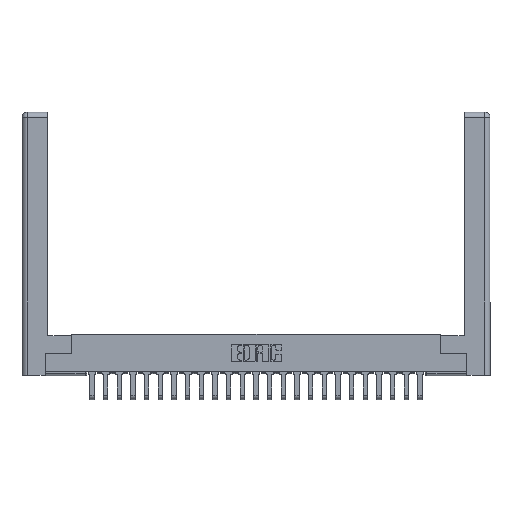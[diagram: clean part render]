
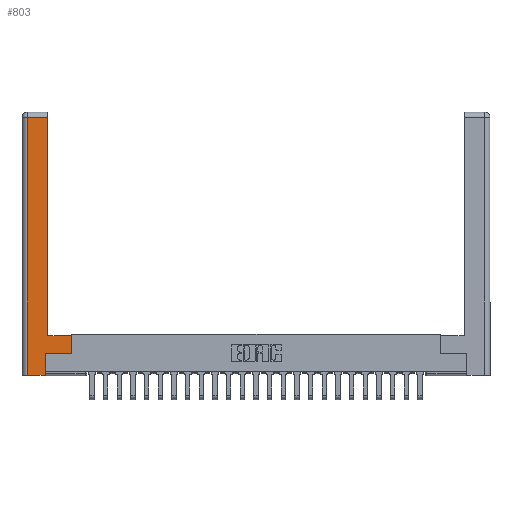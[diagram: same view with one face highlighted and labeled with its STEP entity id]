
A CAD part, top view. The second image highlights one B-rep face of the part: STEP entity #803.
In plain terms, the highlighted planar face has unit normal (0, 0, 1).
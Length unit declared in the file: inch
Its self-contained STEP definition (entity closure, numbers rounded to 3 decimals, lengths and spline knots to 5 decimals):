
#139 = LINE ( 'NONE', #9183, #15880 ) ;
#279 = DIRECTION ( 'NONE',  ( 1., 0., 0. ) ) ;
#803 = ADVANCED_FACE ( 'NONE', ( #17523 ), #23746, .F. ) ;
#818 = CARTESIAN_POINT ( 'NONE',  ( 0.295, 0.45, 0. ) ) ;
#1578 = EDGE_CURVE ( 'NONE', #24801, #14544, #23377, .T. ) ;
#2688 = CARTESIAN_POINT ( 'NONE',  ( 0.565, 0.245, 0. ) ) ;
#2807 = ORIENTED_EDGE ( 'NONE', *, *, #1578, .T. ) ;
#3940 = CARTESIAN_POINT ( 'NONE',  ( 0.0615, 2.94, 0. ) ) ;
#4100 = ORIENTED_EDGE ( 'NONE', *, *, #19604, .T. ) ;
#4155 = CARTESIAN_POINT ( 'NONE',  ( 0.295, 2.94, 0. ) ) ;
#4792 = VERTEX_POINT ( 'NONE', #4155 ) ;
#4798 = VECTOR ( 'NONE', #12545, 39.37008 ) ;
#4860 = DIRECTION ( 'NONE',  ( 0., -1., 0. ) ) ;
#5000 = EDGE_CURVE ( 'NONE', #12074, #17344, #24607, .T. ) ;
#5079 = VECTOR ( 'NONE', #25172, 39.37008 ) ;
#6153 = DIRECTION ( 'NONE',  ( -1., 0., 0. ) ) ;
#6248 = EDGE_CURVE ( 'NONE', #17344, #8954, #139, .T. ) ;
#6306 = ORIENTED_EDGE ( 'NONE', *, *, #8694, .T. ) ;
#6755 = VERTEX_POINT ( 'NONE', #818 ) ;
#7796 = LINE ( 'NONE', #11985, #20072 ) ;
#8694 = EDGE_CURVE ( 'NONE', #4792, #12074, #10130, .T. ) ;
#8954 = VERTEX_POINT ( 'NONE', #11681 ) ;
#8993 = EDGE_LOOP ( 'NONE', ( #12069, #6306, #12452, #15096, #4100, #24421, #2807, #22896 ) ) ;
#9183 = CARTESIAN_POINT ( 'NONE',  ( 0.265, 0., 0. ) ) ;
#10130 = LINE ( 'NONE', #3940, #23446 ) ;
#10365 = EDGE_CURVE ( 'NONE', #14544, #6755, #12393, .T. ) ;
#10383 = CARTESIAN_POINT ( 'NONE',  ( 0.295, 0.45, 0. ) ) ;
#11309 = CARTESIAN_POINT ( 'NONE',  ( 0.565, 0.45, 0. ) ) ;
#11681 = CARTESIAN_POINT ( 'NONE',  ( 0.265, 0., 0. ) ) ;
#11730 = DIRECTION ( 'NONE',  ( 0., 1., 0. ) ) ;
#11985 = CARTESIAN_POINT ( 'NONE',  ( 0.565, 0.245, 0. ) ) ;
#12069 = ORIENTED_EDGE ( 'NONE', *, *, #17331, .T. ) ;
#12074 = VERTEX_POINT ( 'NONE', #13469 ) ;
#12393 = LINE ( 'NONE', #10383, #4798 ) ;
#12452 = ORIENTED_EDGE ( 'NONE', *, *, #5000, .T. ) ;
#12545 = DIRECTION ( 'NONE',  ( -1., 0., 0. ) ) ;
#13469 = CARTESIAN_POINT ( 'NONE',  ( 0.0615, 2.94, 0. ) ) ;
#13739 = LINE ( 'NONE', #18353, #25295 ) ;
#13994 = EDGE_CURVE ( 'NONE', #18421, #24801, #7796, .T. ) ;
#14544 = VERTEX_POINT ( 'NONE', #11309 ) ;
#15096 = ORIENTED_EDGE ( 'NONE', *, *, #6248, .T. ) ;
#15880 = VECTOR ( 'NONE', #279, 39.37008 ) ;
#16377 = CARTESIAN_POINT ( 'NONE',  ( 0.265, 0.245, 0. ) ) ;
#16608 = DIRECTION ( 'NONE',  ( -1., 0., 0. ) ) ;
#17331 = EDGE_CURVE ( 'NONE', #6755, #4792, #13739, .T. ) ;
#17344 = VERTEX_POINT ( 'NONE', #24576 ) ;
#17523 = FACE_OUTER_BOUND ( 'NONE', #8993, .T. ) ;
#18240 = AXIS2_PLACEMENT_3D ( 'NONE', #26178, #24306, #6153 ) ;
#18353 = CARTESIAN_POINT ( 'NONE',  ( 0.295, 3., 0. ) ) ;
#18421 = VERTEX_POINT ( 'NONE', #21136 ) ;
#19604 = EDGE_CURVE ( 'NONE', #8954, #18421, #20857, .T. ) ;
#20072 = VECTOR ( 'NONE', #27824, 39.37008 ) ;
#20857 = LINE ( 'NONE', #16377, #5079 ) ;
#21071 = DIRECTION ( 'NONE',  ( 0., 1., 0. ) ) ;
#21136 = CARTESIAN_POINT ( 'NONE',  ( 0.265, 0.245, 0. ) ) ;
#22896 = ORIENTED_EDGE ( 'NONE', *, *, #10365, .T. ) ;
#23089 = CARTESIAN_POINT ( 'NONE',  ( 0.565, 0.45, 0. ) ) ;
#23377 = LINE ( 'NONE', #23089, #25642 ) ;
#23446 = VECTOR ( 'NONE', #16608, 39.37008 ) ;
#23746 = PLANE ( 'NONE',  #18240 ) ;
#24306 = DIRECTION ( 'NONE',  ( 0., 0., -1. ) ) ;
#24421 = ORIENTED_EDGE ( 'NONE', *, *, #13994, .T. ) ;
#24576 = CARTESIAN_POINT ( 'NONE',  ( 0.0615, 0., 0. ) ) ;
#24607 = LINE ( 'NONE', #26342, #26708 ) ;
#24801 = VERTEX_POINT ( 'NONE', #2688 ) ;
#25172 = DIRECTION ( 'NONE',  ( 0., 1., 0. ) ) ;
#25295 = VECTOR ( 'NONE', #11730, 39.37008 ) ;
#25642 = VECTOR ( 'NONE', #21071, 39.37008 ) ;
#26178 = CARTESIAN_POINT ( 'NONE',  ( 0., 0., 0. ) ) ;
#26342 = CARTESIAN_POINT ( 'NONE',  ( 0.0615, 0., 0. ) ) ;
#26708 = VECTOR ( 'NONE', #4860, 39.37008 ) ;
#27824 = DIRECTION ( 'NONE',  ( 1., 0., 0. ) ) ;
